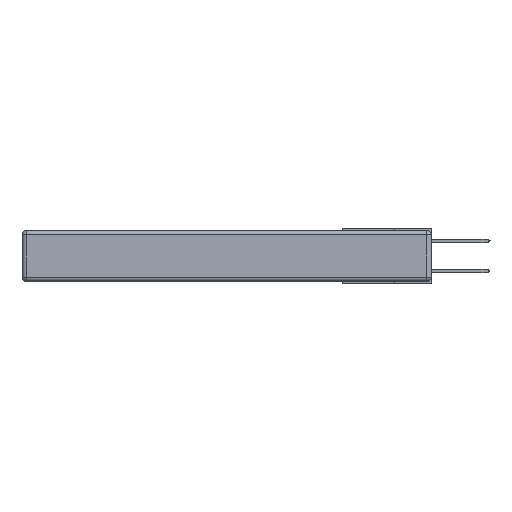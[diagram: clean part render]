
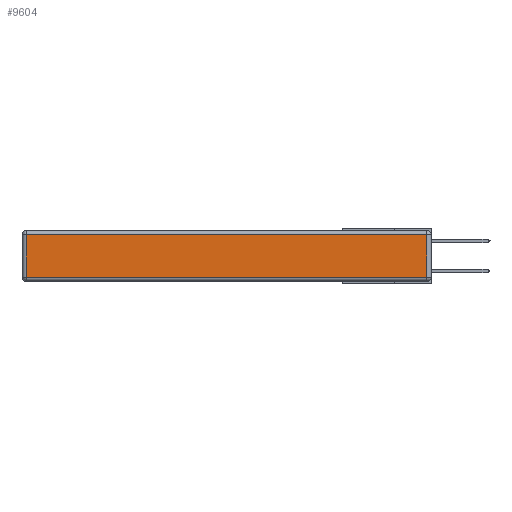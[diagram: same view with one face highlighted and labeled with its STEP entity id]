
A CAD part, left-side view. The second image highlights one B-rep face of the part: STEP entity #9604.
In plain terms, the highlighted planar face has unit normal (-1, 0, 0).
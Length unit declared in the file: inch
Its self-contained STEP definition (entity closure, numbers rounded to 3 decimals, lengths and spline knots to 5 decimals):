
#300 = VECTOR ( 'NONE', #11532, 39.37008 ) ;
#368 = EDGE_CURVE ( 'NONE', #5150, #6611, #3150, .T. ) ;
#651 = EDGE_CURVE ( 'NONE', #7914, #5150, #13040, .T. ) ;
#778 = AXIS2_PLACEMENT_3D ( 'NONE', #11715, #10580, #5000 ) ;
#1513 = EDGE_CURVE ( 'NONE', #11094, #7914, #7212, .T. ) ;
#1988 = VECTOR ( 'NONE', #13226, 39.37008 ) ;
#3150 = LINE ( 'NONE', #5965, #300 ) ;
#4038 = VECTOR ( 'NONE', #5269, 39.37008 ) ;
#5000 = DIRECTION ( 'NONE',  ( 0., 0., 1. ) ) ;
#5150 = VERTEX_POINT ( 'NONE', #12426 ) ;
#5269 = DIRECTION ( 'NONE',  ( 0., -1., 0. ) ) ;
#5406 = DIRECTION ( 'NONE',  ( 0., 0., -1. ) ) ;
#5965 = CARTESIAN_POINT ( 'NONE',  ( 0., 0.03, -0.343 ) ) ;
#6158 = CARTESIAN_POINT ( 'NONE',  ( 0., 2.72, -0.313 ) ) ;
#6316 = CARTESIAN_POINT ( 'NONE',  ( 0., 0., -0.313 ) ) ;
#6611 = VERTEX_POINT ( 'NONE', #8552 ) ;
#7212 = LINE ( 'NONE', #9945, #13029 ) ;
#7914 = VERTEX_POINT ( 'NONE', #6158 ) ;
#8552 = CARTESIAN_POINT ( 'NONE',  ( 0., 0.03, -0.03 ) ) ;
#9604 = ADVANCED_FACE ( 'NONE', ( #13838 ), #12706, .T. ) ;
#9945 = CARTESIAN_POINT ( 'NONE',  ( 0., 2.72, -0.343 ) ) ;
#10328 = ORIENTED_EDGE ( 'NONE', *, *, #651, .T. ) ;
#10580 = DIRECTION ( 'NONE',  ( -1., 0., 0. ) ) ;
#10967 = ORIENTED_EDGE ( 'NONE', *, *, #1513, .T. ) ;
#11094 = VERTEX_POINT ( 'NONE', #12237 ) ;
#11532 = DIRECTION ( 'NONE',  ( 0., 0., 1. ) ) ;
#11625 = EDGE_LOOP ( 'NONE', ( #10328, #12288, #13230, #10967 ) ) ;
#11715 = CARTESIAN_POINT ( 'NONE',  ( 0., 0., -0.343 ) ) ;
#12237 = CARTESIAN_POINT ( 'NONE',  ( 0., 2.72, -0.03 ) ) ;
#12288 = ORIENTED_EDGE ( 'NONE', *, *, #368, .T. ) ;
#12421 = LINE ( 'NONE', #13378, #1988 ) ;
#12426 = CARTESIAN_POINT ( 'NONE',  ( 0., 0.03, -0.313 ) ) ;
#12706 = PLANE ( 'NONE',  #778 ) ;
#13029 = VECTOR ( 'NONE', #5406, 39.37008 ) ;
#13040 = LINE ( 'NONE', #6316, #4038 ) ;
#13226 = DIRECTION ( 'NONE',  ( 0., 1., 0. ) ) ;
#13230 = ORIENTED_EDGE ( 'NONE', *, *, #13901, .T. ) ;
#13378 = CARTESIAN_POINT ( 'NONE',  ( 0., 2.75, -0.03 ) ) ;
#13838 = FACE_OUTER_BOUND ( 'NONE', #11625, .T. ) ;
#13901 = EDGE_CURVE ( 'NONE', #6611, #11094, #12421, .T. ) ;
